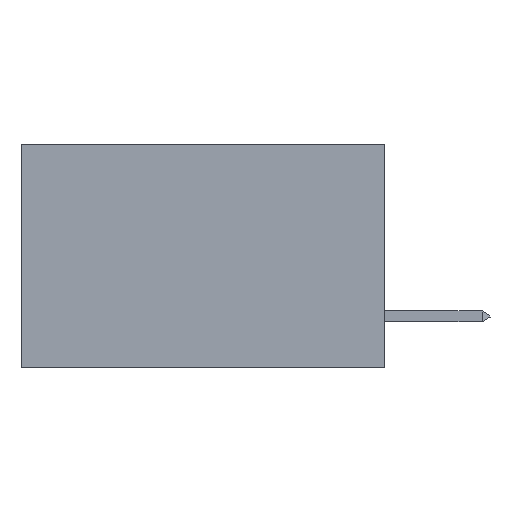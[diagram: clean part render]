
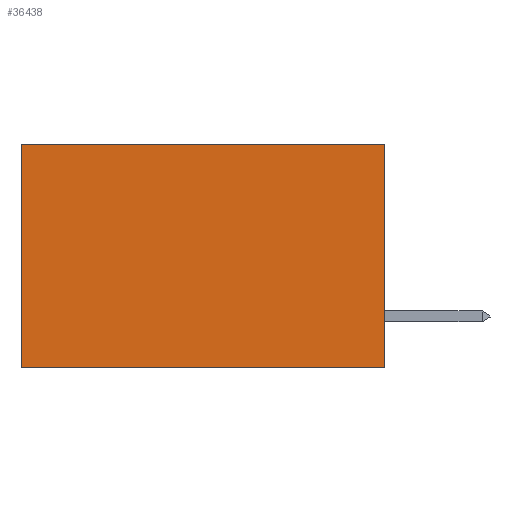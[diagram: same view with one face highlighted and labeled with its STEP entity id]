
A CAD part, left-side view. The second image highlights one B-rep face of the part: STEP entity #36438.
In plain terms, the highlighted planar face has unit normal (-1, 0, 0).
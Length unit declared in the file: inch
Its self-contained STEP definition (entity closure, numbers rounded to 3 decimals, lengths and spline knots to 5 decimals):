
#911 = PLANE ( 'NONE',  #31752 ) ;
#1684 = EDGE_CURVE ( 'NONE', #26542, #37113, #45230, .T. ) ;
#1721 = VECTOR ( 'NONE', #21594, 39.37008 ) ;
#2990 = ORIENTED_EDGE ( 'NONE', *, *, #18837, .T. ) ;
#4844 = VECTOR ( 'NONE', #22892, 39.37008 ) ;
#5039 = EDGE_CURVE ( 'NONE', #18929, #37113, #16367, .T. ) ;
#5735 = ORIENTED_EDGE ( 'NONE', *, *, #1684, .F. ) ;
#8836 = FACE_OUTER_BOUND ( 'NONE', #43068, .T. ) ;
#11188 = EDGE_CURVE ( 'NONE', #42876, #26542, #40631, .T. ) ;
#15083 = DIRECTION ( 'NONE',  ( 1., 0., 0. ) ) ;
#16367 = LINE ( 'NONE', #37510, #4844 ) ;
#17158 = ORIENTED_EDGE ( 'NONE', *, *, #5039, .T. ) ;
#18358 = VECTOR ( 'NONE', #43752, 39.37008 ) ;
#18837 = EDGE_CURVE ( 'NONE', #42876, #18929, #42939, .T. ) ;
#18929 = VERTEX_POINT ( 'NONE', #36657 ) ;
#21594 = DIRECTION ( 'NONE',  ( 0., 1., 0. ) ) ;
#21716 = CARTESIAN_POINT ( 'NONE',  ( 0.2875, 0., -0.37 ) ) ;
#22892 = DIRECTION ( 'NONE',  ( 0., 0., -1. ) ) ;
#23234 = CARTESIAN_POINT ( 'NONE',  ( 0.2875, 0., 0. ) ) ;
#26113 = CARTESIAN_POINT ( 'NONE',  ( 0.2875, 0.6, -0.37 ) ) ;
#26498 = DIRECTION ( 'NONE',  ( 0., 0., -1. ) ) ;
#26542 = VERTEX_POINT ( 'NONE', #40253 ) ;
#28886 = ORIENTED_EDGE ( 'NONE', *, *, #11188, .F. ) ;
#30169 = CARTESIAN_POINT ( 'NONE',  ( 0.2875, 0., 0. ) ) ;
#31752 = AXIS2_PLACEMENT_3D ( 'NONE', #30169, #15083, #26498 ) ;
#34529 = CARTESIAN_POINT ( 'NONE',  ( 0.2875, 0., 0. ) ) ;
#36438 = ADVANCED_FACE ( 'NONE', ( #8836 ), #911, .F. ) ;
#36657 = CARTESIAN_POINT ( 'NONE',  ( 0.2875, 0.6, 0. ) ) ;
#37049 = VECTOR ( 'NONE', #38349, 39.37008 ) ;
#37113 = VERTEX_POINT ( 'NONE', #26113 ) ;
#37510 = CARTESIAN_POINT ( 'NONE',  ( 0.2875, 0.6, 0. ) ) ;
#38349 = DIRECTION ( 'NONE',  ( 0., 0., -1. ) ) ;
#40253 = CARTESIAN_POINT ( 'NONE',  ( 0.2875, 0., -0.37 ) ) ;
#40631 = LINE ( 'NONE', #23234, #37049 ) ;
#42876 = VERTEX_POINT ( 'NONE', #34529 ) ;
#42939 = LINE ( 'NONE', #43477, #1721 ) ;
#43068 = EDGE_LOOP ( 'NONE', ( #17158, #5735, #28886, #2990 ) ) ;
#43477 = CARTESIAN_POINT ( 'NONE',  ( 0.2875, 0., 0. ) ) ;
#43752 = DIRECTION ( 'NONE',  ( 0., 1., 0. ) ) ;
#45230 = LINE ( 'NONE', #21716, #18358 ) ;
